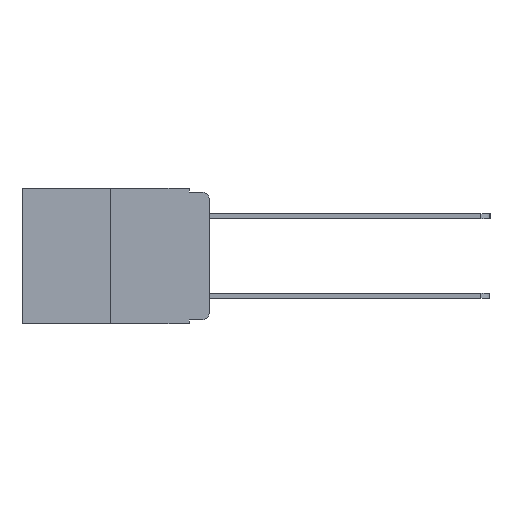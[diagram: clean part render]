
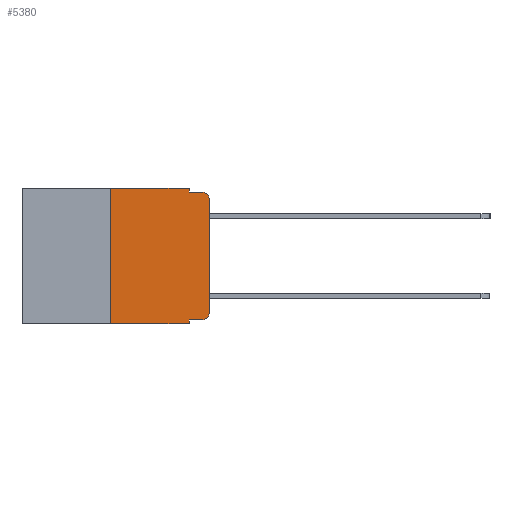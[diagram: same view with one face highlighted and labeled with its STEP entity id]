
A CAD part, left-side view. The second image highlights one B-rep face of the part: STEP entity #5380.
In plain terms, the highlighted planar face has unit normal (-1, 0, 0).
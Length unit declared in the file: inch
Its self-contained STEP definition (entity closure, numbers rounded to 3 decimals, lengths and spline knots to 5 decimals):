
#255 = VERTEX_POINT ( 'NONE', #7295 ) ;
#264 = EDGE_CURVE ( 'NONE', #9735, #7703, #10092, .T. ) ;
#573 = LINE ( 'NONE', #8874, #10039 ) ;
#653 = DIRECTION ( 'NONE',  ( 0., 0., -1. ) ) ;
#826 = CARTESIAN_POINT ( 'NONE',  ( 0., 0.473, 0. ) ) ;
#829 = CARTESIAN_POINT ( 'NONE',  ( 0., 0.051, -0.01 ) ) ;
#1113 = EDGE_CURVE ( 'NONE', #9735, #1748, #5130, .T. ) ;
#1459 = DIRECTION ( 'NONE',  ( 0., -1., 0. ) ) ;
#1748 = VERTEX_POINT ( 'NONE', #3953 ) ;
#1755 = CARTESIAN_POINT ( 'NONE',  ( 0., 0.473, 0. ) ) ;
#2207 = VERTEX_POINT ( 'NONE', #3567 ) ;
#2430 = VERTEX_POINT ( 'NONE', #2948 ) ;
#2443 = LINE ( 'NONE', #8056, #9526 ) ;
#2473 = VECTOR ( 'NONE', #10507, 39.37008 ) ;
#2548 = CARTESIAN_POINT ( 'NONE',  ( 0., 0., 0. ) ) ;
#2760 = PLANE ( 'NONE',  #8731 ) ;
#2948 = CARTESIAN_POINT ( 'NONE',  ( 0., 0., -0.03 ) ) ;
#3042 = VECTOR ( 'NONE', #653, 39.37008 ) ;
#3068 = CARTESIAN_POINT ( 'NONE',  ( 0., 0.051, 0. ) ) ;
#3567 = CARTESIAN_POINT ( 'NONE',  ( 0., 0., -0.313 ) ) ;
#3872 = DIRECTION ( 'NONE',  ( 0., -1., 0. ) ) ;
#3916 = CARTESIAN_POINT ( 'NONE',  ( 0., 0.051, -0.333 ) ) ;
#3918 = VERTEX_POINT ( 'NONE', #10441 ) ;
#3953 = CARTESIAN_POINT ( 'NONE',  ( 0., 0.02, -0.333 ) ) ;
#4065 = VECTOR ( 'NONE', #1459, 39.37008 ) ;
#4070 = CARTESIAN_POINT ( 'NONE',  ( 0., 0.02, -0.03 ) ) ;
#4146 = VERTEX_POINT ( 'NONE', #829 ) ;
#4377 = LINE ( 'NONE', #9688, #2473 ) ;
#4546 = AXIS2_PLACEMENT_3D ( 'NONE', #4070, #10174, #5082 ) ;
#4601 = EDGE_CURVE ( 'NONE', #7289, #4146, #2443, .T. ) ;
#4696 = ORIENTED_EDGE ( 'NONE', *, *, #5253, .F. ) ;
#5082 = DIRECTION ( 'NONE',  ( 0., 0., -1. ) ) ;
#5130 = LINE ( 'NONE', #3916, #9545 ) ;
#5253 = EDGE_CURVE ( 'NONE', #4146, #255, #573, .T. ) ;
#5349 = CARTESIAN_POINT ( 'NONE',  ( 0., 0.051, -0.343 ) ) ;
#5380 = ADVANCED_FACE ( 'NONE', ( #9773 ), #2760, .F. ) ;
#5471 = DIRECTION ( 'NONE',  ( 0., -1., 0. ) ) ;
#5648 = DIRECTION ( 'NONE',  ( 0., 0., -1. ) ) ;
#5805 = CARTESIAN_POINT ( 'NONE',  ( 0., 0.02, -0.313 ) ) ;
#5875 = EDGE_CURVE ( 'NONE', #2207, #2430, #9763, .T. ) ;
#5885 = ORIENTED_EDGE ( 'NONE', *, *, #264, .F. ) ;
#5914 = CARTESIAN_POINT ( 'NONE',  ( 0., 0.25, 0. ) ) ;
#6152 = ORIENTED_EDGE ( 'NONE', *, *, #10689, .T. ) ;
#6220 = CARTESIAN_POINT ( 'NONE',  ( 0., 0.473, -0.343 ) ) ;
#6457 = EDGE_CURVE ( 'NONE', #2430, #255, #10761, .T. ) ;
#6597 = EDGE_LOOP ( 'NONE', ( #6831, #9067, #4696, #7092, #9307, #11678, #10086, #5885, #10333, #6152 ) ) ;
#6632 = DIRECTION ( 'NONE',  ( 0., -1., 0. ) ) ;
#6673 = DIRECTION ( 'NONE',  ( 0., 0., -1. ) ) ;
#6681 = CIRCLE ( 'NONE', #7911, 0.02 ) ;
#6769 = DIRECTION ( 'NONE',  ( 0., 0., -1. ) ) ;
#6831 = ORIENTED_EDGE ( 'NONE', *, *, #5875, .T. ) ;
#7092 = ORIENTED_EDGE ( 'NONE', *, *, #4601, .F. ) ;
#7278 = VERTEX_POINT ( 'NONE', #5914 ) ;
#7289 = VERTEX_POINT ( 'NONE', #3068 ) ;
#7295 = CARTESIAN_POINT ( 'NONE',  ( 0., 0.02, -0.01 ) ) ;
#7703 = VERTEX_POINT ( 'NONE', #5349 ) ;
#7911 = AXIS2_PLACEMENT_3D ( 'NONE', #5805, #11568, #6673 ) ;
#7965 = DIRECTION ( 'NONE',  ( 0., 0., 1. ) ) ;
#8010 = CARTESIAN_POINT ( 'NONE',  ( 0., 0.051, -0.333 ) ) ;
#8056 = CARTESIAN_POINT ( 'NONE',  ( 0., 0.051, 0. ) ) ;
#8402 = CARTESIAN_POINT ( 'NONE',  ( 0., 0.051, 0. ) ) ;
#8731 = AXIS2_PLACEMENT_3D ( 'NONE', #1755, #10635, #5648 ) ;
#8874 = CARTESIAN_POINT ( 'NONE',  ( 0., 0.051, -0.01 ) ) ;
#9067 = ORIENTED_EDGE ( 'NONE', *, *, #6457, .T. ) ;
#9307 = ORIENTED_EDGE ( 'NONE', *, *, #10644, .F. ) ;
#9526 = VECTOR ( 'NONE', #6769, 39.37008 ) ;
#9545 = VECTOR ( 'NONE', #3872, 39.37008 ) ;
#9650 = EDGE_CURVE ( 'NONE', #3918, #7703, #11439, .T. ) ;
#9688 = CARTESIAN_POINT ( 'NONE',  ( 0., 0.25, 0. ) ) ;
#9735 = VERTEX_POINT ( 'NONE', #8010 ) ;
#9763 = LINE ( 'NONE', #2548, #11377 ) ;
#9773 = FACE_OUTER_BOUND ( 'NONE', #6597, .T. ) ;
#10039 = VECTOR ( 'NONE', #5471, 39.37008 ) ;
#10086 = ORIENTED_EDGE ( 'NONE', *, *, #9650, .T. ) ;
#10092 = LINE ( 'NONE', #8402, #3042 ) ;
#10174 = DIRECTION ( 'NONE',  ( -1., 0., 0. ) ) ;
#10333 = ORIENTED_EDGE ( 'NONE', *, *, #1113, .T. ) ;
#10441 = CARTESIAN_POINT ( 'NONE',  ( 0., 0.25, -0.343 ) ) ;
#10507 = DIRECTION ( 'NONE',  ( 0., 0., 1. ) ) ;
#10635 = DIRECTION ( 'NONE',  ( 1., 0., 0. ) ) ;
#10644 = EDGE_CURVE ( 'NONE', #7278, #7289, #11298, .T. ) ;
#10689 = EDGE_CURVE ( 'NONE', #1748, #2207, #6681, .T. ) ;
#10761 = CIRCLE ( 'NONE', #4546, 0.02 ) ;
#11046 = VECTOR ( 'NONE', #6632, 39.37008 ) ;
#11298 = LINE ( 'NONE', #826, #11046 ) ;
#11377 = VECTOR ( 'NONE', #7965, 39.37008 ) ;
#11404 = EDGE_CURVE ( 'NONE', #3918, #7278, #4377, .T. ) ;
#11439 = LINE ( 'NONE', #6220, #4065 ) ;
#11568 = DIRECTION ( 'NONE',  ( -1., 0., 0. ) ) ;
#11678 = ORIENTED_EDGE ( 'NONE', *, *, #11404, .F. ) ;
